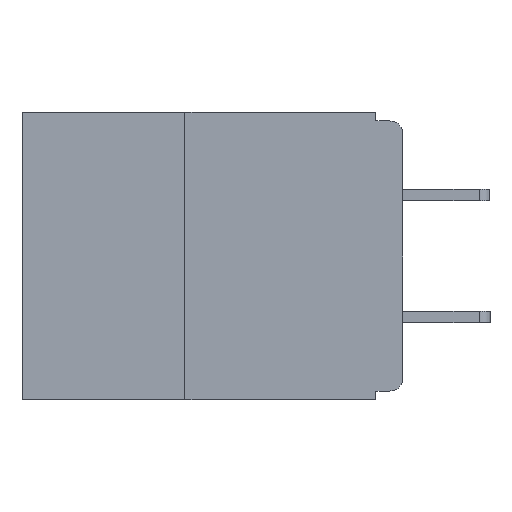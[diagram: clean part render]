
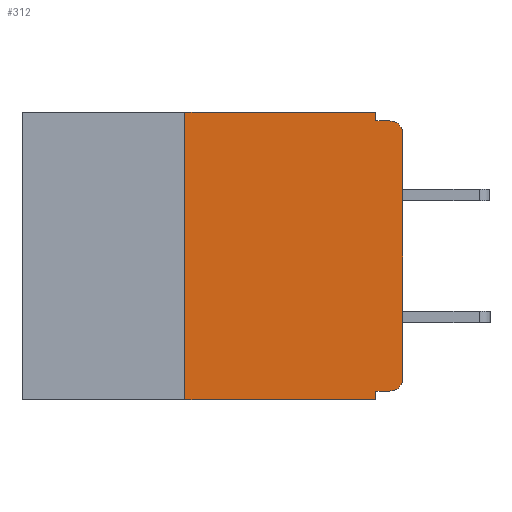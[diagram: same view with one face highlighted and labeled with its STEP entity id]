
A CAD part, left-side view. The second image highlights one B-rep face of the part: STEP entity #312.
In plain terms, the highlighted planar face has unit normal (-1, 0, 0).
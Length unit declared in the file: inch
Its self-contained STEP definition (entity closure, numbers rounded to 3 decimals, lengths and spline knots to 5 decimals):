
#241 = VECTOR ( 'NONE', #2401, 39.37008 ) ;
#267 = CARTESIAN_POINT ( 'NONE',  ( 0., 0.031, 0. ) ) ;
#274 = DIRECTION ( 'NONE',  ( 0., 0., -1. ) ) ;
#312 = ADVANCED_FACE ( 'NONE', ( #18560 ), #16949, .F. ) ;
#470 = CIRCLE ( 'NONE', #15964, 0.015 ) ;
#658 = CARTESIAN_POINT ( 'NONE',  ( 0., 0.25, 0. ) ) ;
#752 = VERTEX_POINT ( 'NONE', #9977 ) ;
#1102 = EDGE_CURVE ( 'NONE', #18416, #17760, #17405, .T. ) ;
#1205 = CIRCLE ( 'NONE', #6779, 0.015 ) ;
#1499 = CARTESIAN_POINT ( 'NONE',  ( 0., 0.031, -0.33 ) ) ;
#1555 = VERTEX_POINT ( 'NONE', #4039 ) ;
#2088 = ORIENTED_EDGE ( 'NONE', *, *, #17828, .T. ) ;
#2300 = CARTESIAN_POINT ( 'NONE',  ( 0., 0.015, -0.305 ) ) ;
#2358 = VERTEX_POINT ( 'NONE', #13933 ) ;
#2401 = DIRECTION ( 'NONE',  ( 0., -1., 0. ) ) ;
#2764 = CARTESIAN_POINT ( 'NONE',  ( 0., 0., -0.01 ) ) ;
#3191 = CARTESIAN_POINT ( 'NONE',  ( 0., 0., 0. ) ) ;
#3868 = EDGE_CURVE ( 'NONE', #2358, #11217, #3943, .T. ) ;
#3943 = LINE ( 'NONE', #10675, #15532 ) ;
#3960 = DIRECTION ( 'NONE',  ( 0., 0., -1. ) ) ;
#4039 = CARTESIAN_POINT ( 'NONE',  ( 0., 0.031, 0. ) ) ;
#4060 = VERTEX_POINT ( 'NONE', #8814 ) ;
#4980 = EDGE_CURVE ( 'NONE', #1555, #13016, #8017, .T. ) ;
#5070 = CARTESIAN_POINT ( 'NONE',  ( 0., 0.031, -0.01 ) ) ;
#5212 = ORIENTED_EDGE ( 'NONE', *, *, #1102, .F. ) ;
#6454 = LINE ( 'NONE', #3191, #13973 ) ;
#6578 = CARTESIAN_POINT ( 'NONE',  ( 0., 0.437, -0.33 ) ) ;
#6779 = AXIS2_PLACEMENT_3D ( 'NONE', #2300, #13173, #3960 ) ;
#6895 = LINE ( 'NONE', #1499, #13934 ) ;
#7160 = DIRECTION ( 'NONE',  ( 0., 1., 0. ) ) ;
#7412 = ORIENTED_EDGE ( 'NONE', *, *, #9666, .F. ) ;
#7637 = CARTESIAN_POINT ( 'NONE',  ( 0., 0.015, -0.025 ) ) ;
#7870 = VERTEX_POINT ( 'NONE', #18804 ) ;
#7946 = VERTEX_POINT ( 'NONE', #15932 ) ;
#8017 = LINE ( 'NONE', #267, #12537 ) ;
#8122 = ORIENTED_EDGE ( 'NONE', *, *, #4980, .F. ) ;
#8466 = DIRECTION ( 'NONE',  ( 0., 0., -1. ) ) ;
#8629 = EDGE_CURVE ( 'NONE', #11217, #1555, #15527, .T. ) ;
#8814 = CARTESIAN_POINT ( 'NONE',  ( 0., 0.031, -0.33 ) ) ;
#8819 = LINE ( 'NONE', #2764, #241 ) ;
#9160 = DIRECTION ( 'NONE',  ( 0., 0., -1. ) ) ;
#9171 = VECTOR ( 'NONE', #7160, 39.37008 ) ;
#9531 = ORIENTED_EDGE ( 'NONE', *, *, #16520, .T. ) ;
#9666 = EDGE_CURVE ( 'NONE', #13016, #752, #8819, .T. ) ;
#9977 = CARTESIAN_POINT ( 'NONE',  ( 0., 0.015, -0.01 ) ) ;
#10038 = ORIENTED_EDGE ( 'NONE', *, *, #8629, .F. ) ;
#10097 = DIRECTION ( 'NONE',  ( 0., -1., 0. ) ) ;
#10547 = CARTESIAN_POINT ( 'NONE',  ( 0., 0.015, -0.32 ) ) ;
#10560 = DIRECTION ( 'NONE',  ( 0., 0., 1. ) ) ;
#10675 = CARTESIAN_POINT ( 'NONE',  ( 0., 0.25, -0.33 ) ) ;
#10890 = CARTESIAN_POINT ( 'NONE',  ( 0., 0.437, 0. ) ) ;
#11132 = VECTOR ( 'NONE', #14372, 39.37008 ) ;
#11217 = VERTEX_POINT ( 'NONE', #658 ) ;
#11297 = DIRECTION ( 'NONE',  ( 1., 0., 0. ) ) ;
#11469 = ORIENTED_EDGE ( 'NONE', *, *, #3868, .F. ) ;
#12031 = CARTESIAN_POINT ( 'NONE',  ( 0., 0.031, -0.32 ) ) ;
#12537 = VECTOR ( 'NONE', #274, 39.37008 ) ;
#13016 = VERTEX_POINT ( 'NONE', #5070 ) ;
#13089 = VECTOR ( 'NONE', #10097, 39.37008 ) ;
#13173 = DIRECTION ( 'NONE',  ( -1., 0., 0. ) ) ;
#13933 = CARTESIAN_POINT ( 'NONE',  ( 0., 0.25, -0.33 ) ) ;
#13934 = VECTOR ( 'NONE', #15360, 39.37008 ) ;
#13973 = VECTOR ( 'NONE', #15354, 39.37008 ) ;
#14111 = AXIS2_PLACEMENT_3D ( 'NONE', #17094, #11297, #8466 ) ;
#14372 = DIRECTION ( 'NONE',  ( 0., -1., 0. ) ) ;
#14960 = EDGE_CURVE ( 'NONE', #18416, #7946, #1205, .T. ) ;
#15354 = DIRECTION ( 'NONE',  ( 0., 0., 1. ) ) ;
#15360 = DIRECTION ( 'NONE',  ( 0., 0., -1. ) ) ;
#15527 = LINE ( 'NONE', #10890, #13089 ) ;
#15532 = VECTOR ( 'NONE', #10560, 39.37008 ) ;
#15735 = ORIENTED_EDGE ( 'NONE', *, *, #19269, .T. ) ;
#15932 = CARTESIAN_POINT ( 'NONE',  ( 0., 0., -0.305 ) ) ;
#15964 = AXIS2_PLACEMENT_3D ( 'NONE', #7637, #17912, #9160 ) ;
#16520 = EDGE_CURVE ( 'NONE', #7946, #7870, #6454, .T. ) ;
#16655 = ORIENTED_EDGE ( 'NONE', *, *, #17340, .F. ) ;
#16949 = PLANE ( 'NONE',  #14111 ) ;
#17094 = CARTESIAN_POINT ( 'NONE',  ( 0., 0.437, 0. ) ) ;
#17340 = EDGE_CURVE ( 'NONE', #17760, #4060, #6895, .T. ) ;
#17405 = LINE ( 'NONE', #19102, #9171 ) ;
#17760 = VERTEX_POINT ( 'NONE', #12031 ) ;
#17828 = EDGE_CURVE ( 'NONE', #7870, #752, #470, .T. ) ;
#17912 = DIRECTION ( 'NONE',  ( -1., 0., 0. ) ) ;
#18004 = ORIENTED_EDGE ( 'NONE', *, *, #14960, .T. ) ;
#18416 = VERTEX_POINT ( 'NONE', #10547 ) ;
#18560 = FACE_OUTER_BOUND ( 'NONE', #18596, .T. ) ;
#18596 = EDGE_LOOP ( 'NONE', ( #9531, #2088, #7412, #8122, #10038, #11469, #15735, #16655, #5212, #18004 ) ) ;
#18804 = CARTESIAN_POINT ( 'NONE',  ( 0., 0., -0.025 ) ) ;
#19102 = CARTESIAN_POINT ( 'NONE',  ( 0., 0., -0.32 ) ) ;
#19269 = EDGE_CURVE ( 'NONE', #2358, #4060, #19672, .T. ) ;
#19672 = LINE ( 'NONE', #6578, #11132 ) ;
